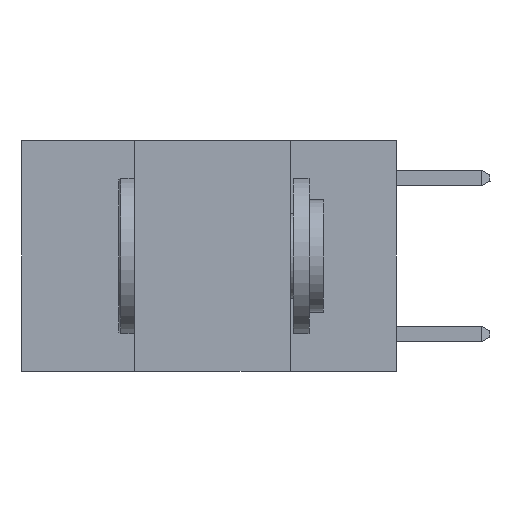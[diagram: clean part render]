
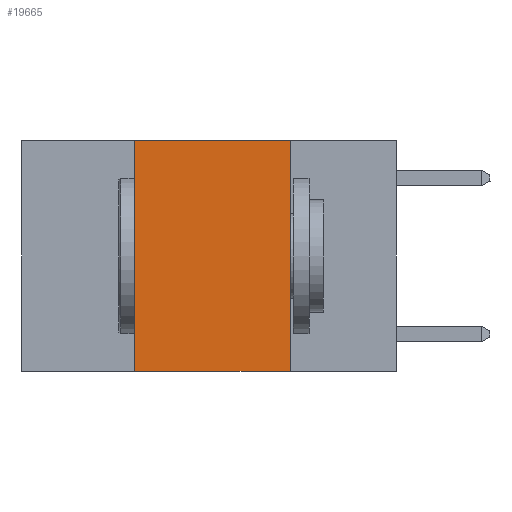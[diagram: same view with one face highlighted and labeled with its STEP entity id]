
A CAD part, left-side view. The second image highlights one B-rep face of the part: STEP entity #19665.
In plain terms, the highlighted planar face has unit normal (-1, 0, 0).
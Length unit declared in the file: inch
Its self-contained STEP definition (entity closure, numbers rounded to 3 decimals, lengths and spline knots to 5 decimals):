
#59 = EDGE_CURVE ( 'NONE', #5154, #9832, #23132, .T. ) ;
#839 = LINE ( 'NONE', #12102, #13918 ) ;
#852 = LINE ( 'NONE', #18787, #25307 ) ;
#1362 = EDGE_CURVE ( 'NONE', #9832, #2515, #839, .T. ) ;
#1804 = ORIENTED_EDGE ( 'NONE', *, *, #1362, .F. ) ;
#2515 = VERTEX_POINT ( 'NONE', #21480 ) ;
#3518 = CARTESIAN_POINT ( 'NONE',  ( 0., 0.42, -0.37 ) ) ;
#4680 = VECTOR ( 'NONE', #24102, 39.37008 ) ;
#4957 = FACE_OUTER_BOUND ( 'NONE', #27013, .T. ) ;
#5154 = VERTEX_POINT ( 'NONE', #5231 ) ;
#5231 = CARTESIAN_POINT ( 'NONE',  ( 0., 0.42, 0. ) ) ;
#5552 = PLANE ( 'NONE',  #9032 ) ;
#6483 = DIRECTION ( 'NONE',  ( 0., -1., 0. ) ) ;
#8028 = DIRECTION ( 'NONE',  ( 0., 0., -1. ) ) ;
#8859 = ORIENTED_EDGE ( 'NONE', *, *, #18063, .F. ) ;
#9032 = AXIS2_PLACEMENT_3D ( 'NONE', #15258, #22608, #8028 ) ;
#9219 = CARTESIAN_POINT ( 'NONE',  ( 0., 0.17, 0. ) ) ;
#9832 = VERTEX_POINT ( 'NONE', #9219 ) ;
#10928 = VECTOR ( 'NONE', #25229, 39.37008 ) ;
#11899 = EDGE_CURVE ( 'NONE', #24446, #2515, #852, .T. ) ;
#12102 = CARTESIAN_POINT ( 'NONE',  ( 0., 0.17, 0. ) ) ;
#13918 = VECTOR ( 'NONE', #14558, 39.37008 ) ;
#14558 = DIRECTION ( 'NONE',  ( 0., 0., -1. ) ) ;
#15258 = CARTESIAN_POINT ( 'NONE',  ( 0., 0.6, 0. ) ) ;
#17530 = ORIENTED_EDGE ( 'NONE', *, *, #11899, .T. ) ;
#18063 = EDGE_CURVE ( 'NONE', #24446, #5154, #31089, .T. ) ;
#18787 = CARTESIAN_POINT ( 'NONE',  ( 0., 0.6, -0.37 ) ) ;
#19172 = ORIENTED_EDGE ( 'NONE', *, *, #59, .F. ) ;
#19665 = ADVANCED_FACE ( 'NONE', ( #4957 ), #5552, .F. ) ;
#21480 = CARTESIAN_POINT ( 'NONE',  ( 0., 0.17, -0.37 ) ) ;
#22608 = DIRECTION ( 'NONE',  ( 1., 0., 0. ) ) ;
#23132 = LINE ( 'NONE', #25560, #10928 ) ;
#24102 = DIRECTION ( 'NONE',  ( 0., 0., 1. ) ) ;
#24446 = VERTEX_POINT ( 'NONE', #3518 ) ;
#25229 = DIRECTION ( 'NONE',  ( 0., -1., 0. ) ) ;
#25307 = VECTOR ( 'NONE', #6483, 39.37008 ) ;
#25560 = CARTESIAN_POINT ( 'NONE',  ( 0., 0.6, 0. ) ) ;
#27013 = EDGE_LOOP ( 'NONE', ( #1804, #19172, #8859, #17530 ) ) ;
#31086 = CARTESIAN_POINT ( 'NONE',  ( 0., 0.42, 0. ) ) ;
#31089 = LINE ( 'NONE', #31086, #4680 ) ;
